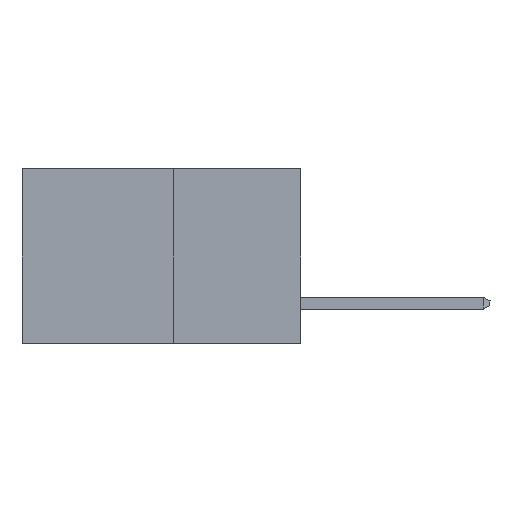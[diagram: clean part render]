
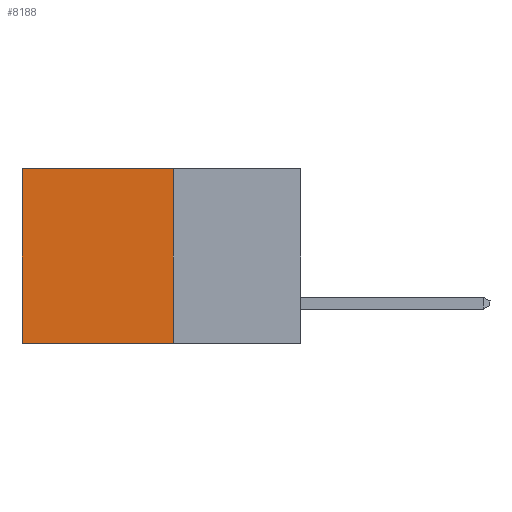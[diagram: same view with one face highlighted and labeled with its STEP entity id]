
A CAD part, left-side view. The second image highlights one B-rep face of the part: STEP entity #8188.
In plain terms, the highlighted planar face has unit normal (-1, 0, 0).
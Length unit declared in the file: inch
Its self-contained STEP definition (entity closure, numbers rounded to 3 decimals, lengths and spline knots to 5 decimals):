
#190 = CARTESIAN_POINT ( 'NONE',  ( 0.277, 0.59, -0.37 ) ) ;
#1809 = ORIENTED_EDGE ( 'NONE', *, *, #10658, .F. ) ;
#1877 = EDGE_CURVE ( 'NONE', #7864, #16381, #15503, .T. ) ;
#2141 = CARTESIAN_POINT ( 'NONE',  ( 0.277, 0.27, 0. ) ) ;
#3241 = VECTOR ( 'NONE', #18704, 39.37008 ) ;
#3552 = DIRECTION ( 'NONE',  ( 0., 0., -1. ) ) ;
#3653 = VERTEX_POINT ( 'NONE', #11265 ) ;
#4471 = VERTEX_POINT ( 'NONE', #21014 ) ;
#6257 = ORIENTED_EDGE ( 'NONE', *, *, #13027, .T. ) ;
#6396 = PLANE ( 'NONE',  #21117 ) ;
#7385 = ORIENTED_EDGE ( 'NONE', *, *, #1877, .F. ) ;
#7864 = VERTEX_POINT ( 'NONE', #20340 ) ;
#8188 = ADVANCED_FACE ( 'NONE', ( #14306 ), #6396, .F. ) ;
#8851 = DIRECTION ( 'NONE',  ( 0., 1., 0. ) ) ;
#10038 = LINE ( 'NONE', #2141, #14384 ) ;
#10658 = EDGE_CURVE ( 'NONE', #16381, #4471, #16524, .T. ) ;
#11140 = VECTOR ( 'NONE', #15764, 39.37008 ) ;
#11265 = CARTESIAN_POINT ( 'NONE',  ( 0.277, 0.59, 0. ) ) ;
#11403 = CARTESIAN_POINT ( 'NONE',  ( 0.277, 0.27, -0.37 ) ) ;
#11475 = DIRECTION ( 'NONE',  ( 0., 0., -1. ) ) ;
#12359 = VECTOR ( 'NONE', #3552, 39.37008 ) ;
#13027 = EDGE_CURVE ( 'NONE', #3653, #4471, #21433, .T. ) ;
#13767 = CARTESIAN_POINT ( 'NONE',  ( 0.277, 0.27, -0.37 ) ) ;
#14306 = FACE_OUTER_BOUND ( 'NONE', #17697, .T. ) ;
#14384 = VECTOR ( 'NONE', #8851, 39.37008 ) ;
#14398 = CARTESIAN_POINT ( 'NONE',  ( 0.277, 0.27, -0.37 ) ) ;
#15503 = LINE ( 'NONE', #14398, #11140 ) ;
#15764 = DIRECTION ( 'NONE',  ( 0., 0., -1. ) ) ;
#16381 = VERTEX_POINT ( 'NONE', #13767 ) ;
#16524 = LINE ( 'NONE', #17082, #3241 ) ;
#16959 = EDGE_CURVE ( 'NONE', #7864, #3653, #10038, .T. ) ;
#17082 = CARTESIAN_POINT ( 'NONE',  ( 0.277, 0.27, -0.37 ) ) ;
#17697 = EDGE_LOOP ( 'NONE', ( #6257, #1809, #7385, #19453 ) ) ;
#18704 = DIRECTION ( 'NONE',  ( 0., 1., 0. ) ) ;
#19453 = ORIENTED_EDGE ( 'NONE', *, *, #16959, .T. ) ;
#20340 = CARTESIAN_POINT ( 'NONE',  ( 0.277, 0.27, 0. ) ) ;
#21014 = CARTESIAN_POINT ( 'NONE',  ( 0.277, 0.59, -0.37 ) ) ;
#21117 = AXIS2_PLACEMENT_3D ( 'NONE', #11403, #21158, #11475 ) ;
#21158 = DIRECTION ( 'NONE',  ( 1., 0., 0. ) ) ;
#21433 = LINE ( 'NONE', #190, #12359 ) ;
